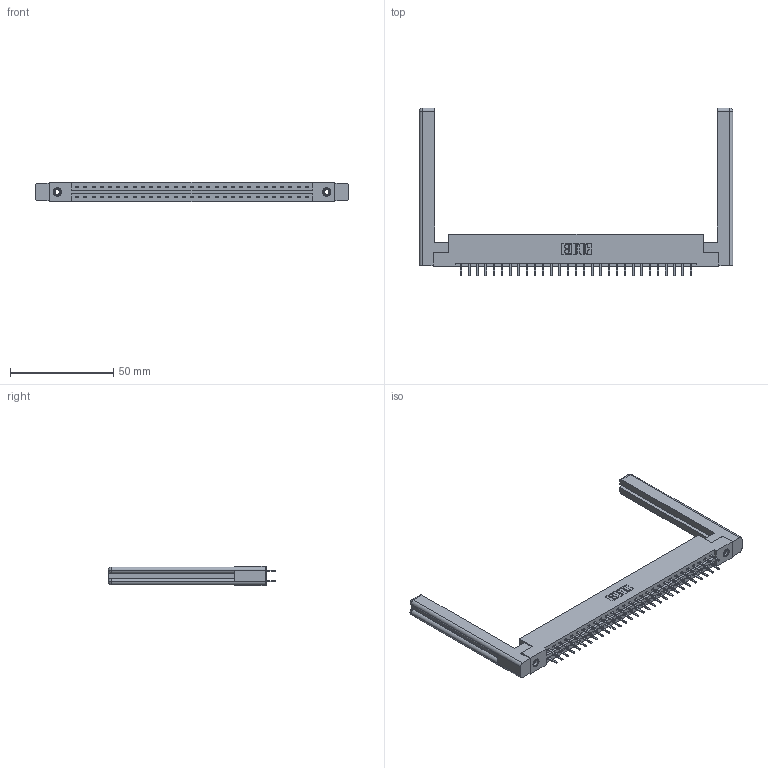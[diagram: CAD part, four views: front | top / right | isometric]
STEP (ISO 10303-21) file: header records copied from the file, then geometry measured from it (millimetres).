
FILE_DESCRIPTION (( 'STEP AP203' ), '1' );
FILE_NAME ('337-058-520-258.STEP', '2019-10-09T19:30:08', ( '' ), ( '' ), 'SwSTEP 2.0', 'SolidWorks 2016', '' );
FILE_SCHEMA (( 'CONFIG_CONTROL_DESIGN' ));
Length unit declared in the file: inch
Products named in the file (5): 345-250-001_345-250-001-102; 307-220-058; 345-292-001_345-293-120; 337 Part_Flush Mounting Lugs - 0.156 Dia-TI; 337-058-520-258
Assembly tree (63 placements, depth 2):
  337-058-520-258
    337 Part_Flush Mounting Lugs - 0.156 Dia-TI
    345-292-001_345-293-120  x58
    345-250-001_345-250-001-102  x2
    307-220-058  x2
Bounding box: 151.54 x 81.11 x 9.4 mm (x, y, z)
Volume: 22913.9 mm3; surface area: 22677.5 mm2
Topology: 63 solids, 63 shells, 3620 faces, 10467 edges, 6810 vertices
Faces by surface type: plane 2474, cylinder 1122, cone 12, torus 12
Entity records: 26914 total; most frequent: CARTESIAN_POINT 4565, ORIENTED_EDGE 4428, DIRECTION 3910, EDGE_CURVE 2214, LINE 2034, VECTOR 2034, VERTEX_POINT 1466, AXIS2_PLACEMENT_3D 938
